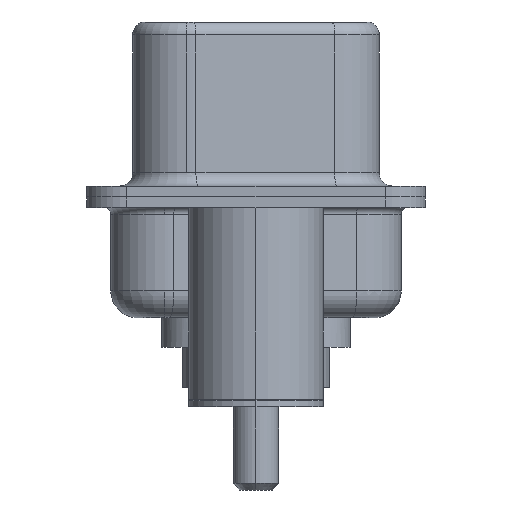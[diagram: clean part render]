
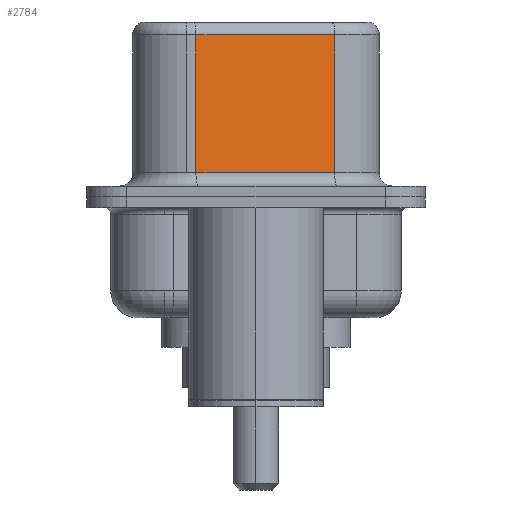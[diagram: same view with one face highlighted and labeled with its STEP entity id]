
A CAD part, left-side view. The second image highlights one B-rep face of the part: STEP entity #2784.
In plain terms, the highlighted planar face has unit normal (-0.985, -0.174, 0).
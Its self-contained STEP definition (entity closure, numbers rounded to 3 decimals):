
#136 = EDGE_CURVE ( 'NONE', #5434, #656, #5592, .T. ) ;
#656 = VERTEX_POINT ( 'NONE', #12011 ) ;
#813 = DIRECTION ( 'NONE',  ( 0.985, 0.174, 0. ) ) ;
#2176 = FACE_OUTER_BOUND ( 'NONE', #6285, .T. ) ;
#2416 = VECTOR ( 'NONE', #3922, 1000. ) ;
#2569 = CARTESIAN_POINT ( 'NONE',  ( 4.585, -2.927, 6.02 ) ) ;
#2784 = ADVANCED_FACE ( 'NONE', ( #2176 ), #6083, .F. ) ;
#3454 = ORIENTED_EDGE ( 'NONE', *, *, #8699, .T. ) ;
#3495 = DIRECTION ( 'NONE',  ( 0., 0., -1. ) ) ;
#3497 = VECTOR ( 'NONE', #7258, 1000. ) ;
#3524 = ORIENTED_EDGE ( 'NONE', *, *, #136, .T. ) ;
#3643 = ORIENTED_EDGE ( 'NONE', *, *, #6196, .T. ) ;
#3760 = ORIENTED_EDGE ( 'NONE', *, *, #8678, .F. ) ;
#3922 = DIRECTION ( 'NONE',  ( 0., 0., -1. ) ) ;
#4506 = LINE ( 'NONE', #10826, #10622 ) ;
#5141 = CARTESIAN_POINT ( 'NONE',  ( 4.585, -2.927, 6.52 ) ) ;
#5180 = CARTESIAN_POINT ( 'NONE',  ( 3.675, 2.233, 6.52 ) ) ;
#5434 = VERTEX_POINT ( 'NONE', #14690 ) ;
#5592 = LINE ( 'NONE', #5180, #2416 ) ;
#6083 = PLANE ( 'NONE',  #14315 ) ;
#6196 = EDGE_CURVE ( 'NONE', #11130, #5434, #4506, .T. ) ;
#6285 = EDGE_LOOP ( 'NONE', ( #3760, #3643, #3524, #3454 ) ) ;
#6567 = DIRECTION ( 'NONE',  ( -0.174, 0.985, 0. ) ) ;
#7258 = DIRECTION ( 'NONE',  ( 0.174, -0.985, 0. ) ) ;
#7341 = DIRECTION ( 'NONE',  ( -0.174, 0.985, 0. ) ) ;
#7700 = VECTOR ( 'NONE', #3495, 1000. ) ;
#8497 = CARTESIAN_POINT ( 'NONE',  ( 4.585, -2.927, 0.9 ) ) ;
#8678 = EDGE_CURVE ( 'NONE', #11130, #9335, #13725, .T. ) ;
#8699 = EDGE_CURVE ( 'NONE', #656, #9335, #12667, .T. ) ;
#9335 = VERTEX_POINT ( 'NONE', #8497 ) ;
#10415 = CARTESIAN_POINT ( 'NONE',  ( 4.585, -2.927, 6.52 ) ) ;
#10622 = VECTOR ( 'NONE', #7341, 1000. ) ;
#10826 = CARTESIAN_POINT ( 'NONE',  ( 4.585, -2.927, 6.02 ) ) ;
#11130 = VERTEX_POINT ( 'NONE', #2569 ) ;
#12011 = CARTESIAN_POINT ( 'NONE',  ( 3.675, 2.233, 0.9 ) ) ;
#12667 = LINE ( 'NONE', #12921, #3497 ) ;
#12921 = CARTESIAN_POINT ( 'NONE',  ( 4.585, -2.927, 0.9 ) ) ;
#13725 = LINE ( 'NONE', #10415, #7700 ) ;
#14315 = AXIS2_PLACEMENT_3D ( 'NONE', #5141, #813, #6567 ) ;
#14690 = CARTESIAN_POINT ( 'NONE',  ( 3.675, 2.233, 6.02 ) ) ;
